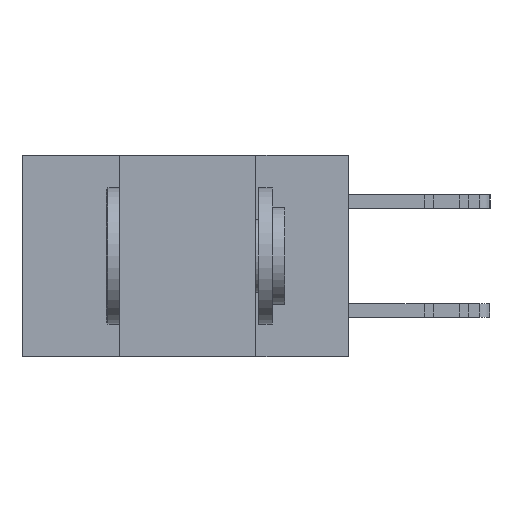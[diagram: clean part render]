
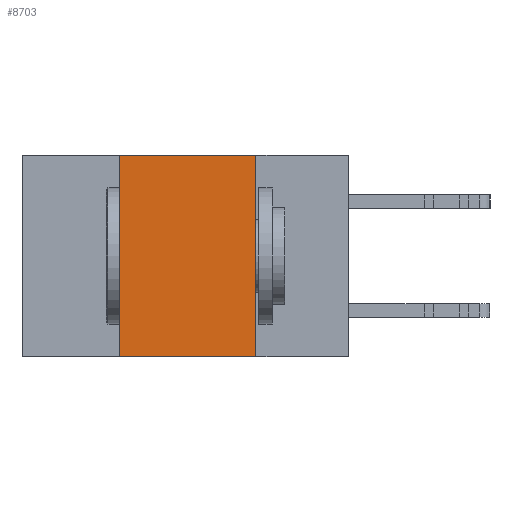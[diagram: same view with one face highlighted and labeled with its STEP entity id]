
A CAD part, left-side view. The second image highlights one B-rep face of the part: STEP entity #8703.
In plain terms, the highlighted planar face has unit normal (-1, 0, 0).
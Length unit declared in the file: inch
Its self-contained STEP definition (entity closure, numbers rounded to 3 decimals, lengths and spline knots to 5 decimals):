
#616 = DIRECTION ( 'NONE',  ( 1., 0., 0. ) ) ;
#779 = ORIENTED_EDGE ( 'NONE', *, *, #18475, .F. ) ;
#1048 = VERTEX_POINT ( 'NONE', #12073 ) ;
#1397 = DIRECTION ( 'NONE',  ( 0., 0., 1. ) ) ;
#3223 = VERTEX_POINT ( 'NONE', #18618 ) ;
#3880 = DIRECTION ( 'NONE',  ( 0., -1., 0. ) ) ;
#5158 = VECTOR ( 'NONE', #15300, 39.37008 ) ;
#5736 = LINE ( 'NONE', #26300, #24056 ) ;
#6038 = VERTEX_POINT ( 'NONE', #12287 ) ;
#6182 = ORIENTED_EDGE ( 'NONE', *, *, #6208, .T. ) ;
#6208 = EDGE_CURVE ( 'NONE', #3223, #6038, #21737, .T. ) ;
#7564 = EDGE_CURVE ( 'NONE', #3223, #1048, #5736, .T. ) ;
#8703 = ADVANCED_FACE ( 'NONE', ( #21057 ), #25254, .F. ) ;
#8800 = ORIENTED_EDGE ( 'NONE', *, *, #12145, .F. ) ;
#11109 = CARTESIAN_POINT ( 'NONE',  ( 0., 0.17, -0.37 ) ) ;
#11150 = AXIS2_PLACEMENT_3D ( 'NONE', #19171, #616, #17134 ) ;
#12073 = CARTESIAN_POINT ( 'NONE',  ( 0., 0.42, 0. ) ) ;
#12145 = EDGE_CURVE ( 'NONE', #19756, #6038, #23690, .T. ) ;
#12287 = CARTESIAN_POINT ( 'NONE',  ( 0., 0.17, -0.37 ) ) ;
#15300 = DIRECTION ( 'NONE',  ( 0., 0., -1. ) ) ;
#16304 = LINE ( 'NONE', #24156, #19166 ) ;
#16647 = CARTESIAN_POINT ( 'NONE',  ( 0., 0.17, 0. ) ) ;
#17134 = DIRECTION ( 'NONE',  ( 0., 0., -1. ) ) ;
#18475 = EDGE_CURVE ( 'NONE', #1048, #19756, #16304, .T. ) ;
#18618 = CARTESIAN_POINT ( 'NONE',  ( 0., 0.42, -0.37 ) ) ;
#19166 = VECTOR ( 'NONE', #3880, 39.37008 ) ;
#19171 = CARTESIAN_POINT ( 'NONE',  ( 0., 0.6, 0. ) ) ;
#19756 = VERTEX_POINT ( 'NONE', #16647 ) ;
#21057 = FACE_OUTER_BOUND ( 'NONE', #22819, .T. ) ;
#21737 = LINE ( 'NONE', #24153, #22140 ) ;
#22115 = DIRECTION ( 'NONE',  ( 0., -1., 0. ) ) ;
#22140 = VECTOR ( 'NONE', #22115, 39.37008 ) ;
#22819 = EDGE_LOOP ( 'NONE', ( #8800, #779, #23325, #6182 ) ) ;
#23325 = ORIENTED_EDGE ( 'NONE', *, *, #7564, .F. ) ;
#23690 = LINE ( 'NONE', #11109, #5158 ) ;
#24056 = VECTOR ( 'NONE', #1397, 39.37008 ) ;
#24153 = CARTESIAN_POINT ( 'NONE',  ( 0., 0.6, -0.37 ) ) ;
#24156 = CARTESIAN_POINT ( 'NONE',  ( 0., 0.6, 0. ) ) ;
#25254 = PLANE ( 'NONE',  #11150 ) ;
#26300 = CARTESIAN_POINT ( 'NONE',  ( 0., 0.42, -0.37 ) ) ;
